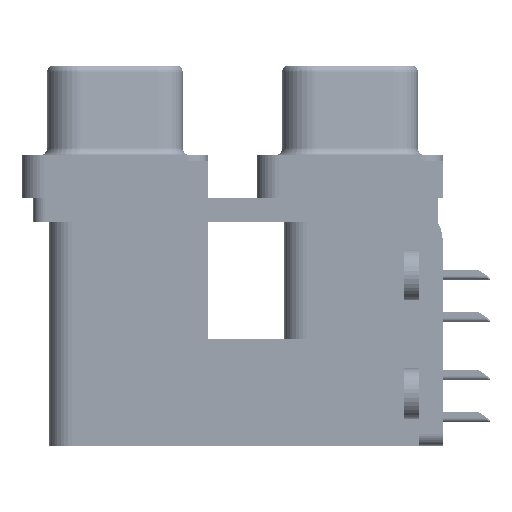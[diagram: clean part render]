
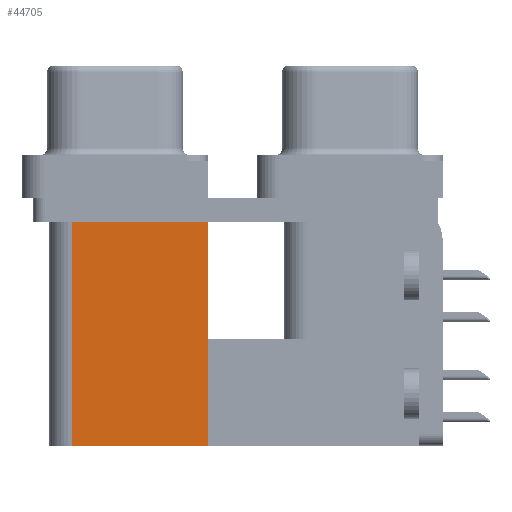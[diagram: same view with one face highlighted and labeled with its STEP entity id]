
A CAD part, left-side view. The second image highlights one B-rep face of the part: STEP entity #44705.
In plain terms, the highlighted planar face has unit normal (-1, 0, 0).
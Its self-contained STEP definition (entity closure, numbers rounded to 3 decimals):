
#62 = ORIENTED_EDGE ( 'NONE', *, *, #5903, .T. ) ;
#4487 = CARTESIAN_POINT ( 'NONE',  ( 3.79, 9.6, -19.2 ) ) ;
#5675 = AXIS2_PLACEMENT_3D ( 'NONE', #29716, #9247, #42097 ) ;
#5861 = CARTESIAN_POINT ( 'NONE',  ( 3.79, 9.6, -19.2 ) ) ;
#5903 = EDGE_CURVE ( 'NONE', #31987, #17912, #19227, .T. ) ;
#9223 = CARTESIAN_POINT ( 'NONE',  ( 3.79, 9.6, -2.5 ) ) ;
#9247 = DIRECTION ( 'NONE',  ( 1., 0., 0. ) ) ;
#9693 = EDGE_CURVE ( 'NONE', #52583, #18703, #47268, .T. ) ;
#11414 = EDGE_CURVE ( 'NONE', #31987, #52583, #41613, .T. ) ;
#13875 = CARTESIAN_POINT ( 'NONE',  ( 3.79, 18.8, -19.2 ) ) ;
#15703 = CARTESIAN_POINT ( 'NONE',  ( 3.79, 18.8, -19.2 ) ) ;
#17912 = VERTEX_POINT ( 'NONE', #37588 ) ;
#18703 = VERTEX_POINT ( 'NONE', #20287 ) ;
#19227 = LINE ( 'NONE', #35616, #21323 ) ;
#19330 = EDGE_CURVE ( 'NONE', #17912, #18703, #26701, .T. ) ;
#20287 = CARTESIAN_POINT ( 'NONE',  ( 3.79, 18.8, -2.5 ) ) ;
#21323 = VECTOR ( 'NONE', #52078, 1000. ) ;
#26195 = DIRECTION ( 'NONE',  ( 0., 1., 0. ) ) ;
#26701 = LINE ( 'NONE', #9223, #42286 ) ;
#29220 = VECTOR ( 'NONE', #33815, 1000. ) ;
#29716 = CARTESIAN_POINT ( 'NONE',  ( 3.79, 9.6, -19.2 ) ) ;
#30985 = ORIENTED_EDGE ( 'NONE', *, *, #9693, .F. ) ;
#31987 = VERTEX_POINT ( 'NONE', #5861 ) ;
#33815 = DIRECTION ( 'NONE',  ( 0., 1., 0. ) ) ;
#35616 = CARTESIAN_POINT ( 'NONE',  ( 3.79, 9.6, -19.2 ) ) ;
#37160 = ORIENTED_EDGE ( 'NONE', *, *, #19330, .T. ) ;
#37588 = CARTESIAN_POINT ( 'NONE',  ( 3.79, 9.6, -2.5 ) ) ;
#41613 = LINE ( 'NONE', #4487, #29220 ) ;
#42097 = DIRECTION ( 'NONE',  ( 0., 0., -1. ) ) ;
#42286 = VECTOR ( 'NONE', #26195, 1000. ) ;
#42419 = DIRECTION ( 'NONE',  ( 0., 0., 1. ) ) ;
#42882 = EDGE_LOOP ( 'NONE', ( #37160, #30985, #47414, #62 ) ) ;
#44705 = ADVANCED_FACE ( 'NONE', ( #50207 ), #50748, .F. ) ;
#47268 = LINE ( 'NONE', #13875, #52715 ) ;
#47414 = ORIENTED_EDGE ( 'NONE', *, *, #11414, .F. ) ;
#50207 = FACE_OUTER_BOUND ( 'NONE', #42882, .T. ) ;
#50748 = PLANE ( 'NONE',  #5675 ) ;
#52078 = DIRECTION ( 'NONE',  ( 0., 0., 1. ) ) ;
#52583 = VERTEX_POINT ( 'NONE', #15703 ) ;
#52715 = VECTOR ( 'NONE', #42419, 1000. ) ;
